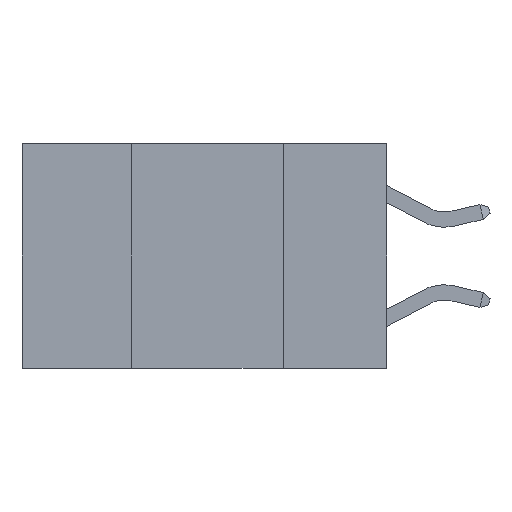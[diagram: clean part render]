
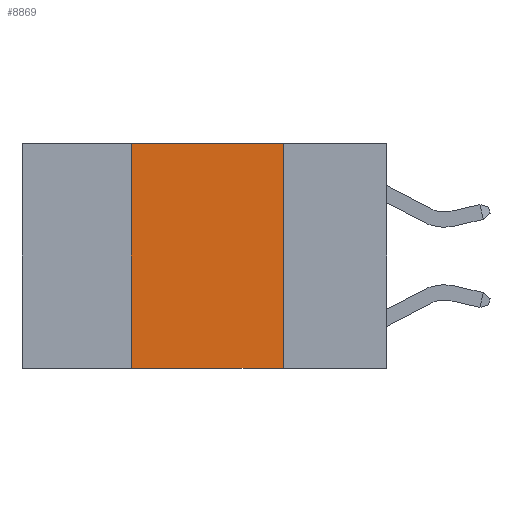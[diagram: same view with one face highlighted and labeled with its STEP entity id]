
A CAD part, left-side view. The second image highlights one B-rep face of the part: STEP entity #8869.
In plain terms, the highlighted planar face has unit normal (-1, 0, 0).
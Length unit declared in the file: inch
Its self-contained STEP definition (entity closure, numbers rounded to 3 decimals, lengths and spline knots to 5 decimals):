
#290 = VECTOR ( 'NONE', #5021, 39.37008 ) ;
#521 = AXIS2_PLACEMENT_3D ( 'NONE', #2960, #6746, #2016 ) ;
#748 = ORIENTED_EDGE ( 'NONE', *, *, #5009, .F. ) ;
#824 = CARTESIAN_POINT ( 'NONE',  ( 0., 0.42, 0. ) ) ;
#1636 = CARTESIAN_POINT ( 'NONE',  ( 0., 0.42, -0.37 ) ) ;
#2016 = DIRECTION ( 'NONE',  ( 0., 0., -1. ) ) ;
#2883 = ORIENTED_EDGE ( 'NONE', *, *, #5298, .F. ) ;
#2960 = CARTESIAN_POINT ( 'NONE',  ( 0., 0.6, 0. ) ) ;
#3110 = CARTESIAN_POINT ( 'NONE',  ( 0., 0.6, 0. ) ) ;
#4522 = ORIENTED_EDGE ( 'NONE', *, *, #11057, .F. ) ;
#4525 = DIRECTION ( 'NONE',  ( 0., 0., 1. ) ) ;
#5009 = EDGE_CURVE ( 'NONE', #5826, #9939, #8096, .T. ) ;
#5021 = DIRECTION ( 'NONE',  ( 0., -1., 0. ) ) ;
#5115 = LINE ( 'NONE', #10127, #10302 ) ;
#5298 = EDGE_CURVE ( 'NONE', #12011, #5826, #10103, .T. ) ;
#5654 = EDGE_CURVE ( 'NONE', #12011, #8633, #6037, .T. ) ;
#5826 = VERTEX_POINT ( 'NONE', #9070 ) ;
#5840 = VECTOR ( 'NONE', #4525, 39.37008 ) ;
#6037 = LINE ( 'NONE', #9783, #290 ) ;
#6746 = DIRECTION ( 'NONE',  ( 1., 0., 0. ) ) ;
#6871 = FACE_OUTER_BOUND ( 'NONE', #9000, .T. ) ;
#7040 = CARTESIAN_POINT ( 'NONE',  ( 0., 0.17, -0.37 ) ) ;
#7415 = VECTOR ( 'NONE', #11427, 39.37008 ) ;
#8096 = LINE ( 'NONE', #3110, #7415 ) ;
#8582 = PLANE ( 'NONE',  #521 ) ;
#8633 = VERTEX_POINT ( 'NONE', #7040 ) ;
#8869 = ADVANCED_FACE ( 'NONE', ( #6871 ), #8582, .F. ) ;
#9000 = EDGE_LOOP ( 'NONE', ( #4522, #748, #2883, #11370 ) ) ;
#9070 = CARTESIAN_POINT ( 'NONE',  ( 0., 0.42, 0. ) ) ;
#9495 = CARTESIAN_POINT ( 'NONE',  ( 0., 0.17, 0. ) ) ;
#9783 = CARTESIAN_POINT ( 'NONE',  ( 0., 0.6, -0.37 ) ) ;
#9939 = VERTEX_POINT ( 'NONE', #9495 ) ;
#10063 = DIRECTION ( 'NONE',  ( 0., 0., -1. ) ) ;
#10103 = LINE ( 'NONE', #824, #5840 ) ;
#10127 = CARTESIAN_POINT ( 'NONE',  ( 0., 0.17, 0. ) ) ;
#10302 = VECTOR ( 'NONE', #10063, 39.37008 ) ;
#11057 = EDGE_CURVE ( 'NONE', #9939, #8633, #5115, .T. ) ;
#11370 = ORIENTED_EDGE ( 'NONE', *, *, #5654, .T. ) ;
#11427 = DIRECTION ( 'NONE',  ( 0., -1., 0. ) ) ;
#12011 = VERTEX_POINT ( 'NONE', #1636 ) ;
